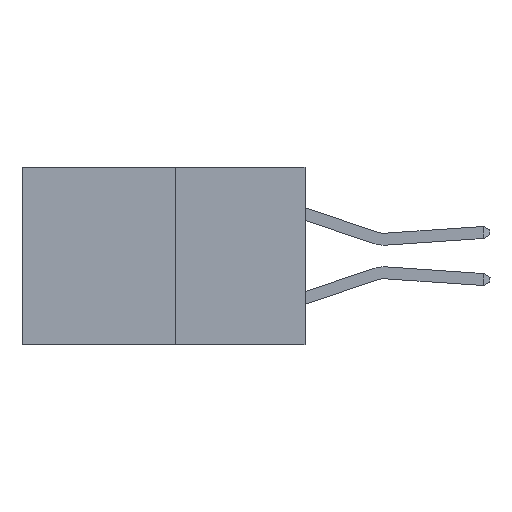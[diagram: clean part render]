
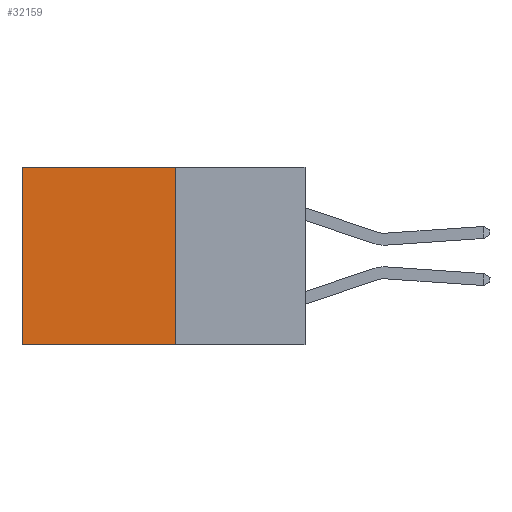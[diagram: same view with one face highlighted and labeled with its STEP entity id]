
A CAD part, left-side view. The second image highlights one B-rep face of the part: STEP entity #32159.
In plain terms, the highlighted planar face has unit normal (-1, 0, 0).
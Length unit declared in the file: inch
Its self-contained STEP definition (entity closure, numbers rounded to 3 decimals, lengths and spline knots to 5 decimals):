
#312 = EDGE_CURVE ( 'NONE', #10957, #1401, #4505, .T. ) ;
#1401 = VERTEX_POINT ( 'NONE', #15070 ) ;
#2053 = ORIENTED_EDGE ( 'NONE', *, *, #21790, .T. ) ;
#2580 = VECTOR ( 'NONE', #31204, 39.37008 ) ;
#4337 = LINE ( 'NONE', #11667, #10253 ) ;
#4505 = LINE ( 'NONE', #17044, #10426 ) ;
#4936 = VERTEX_POINT ( 'NONE', #7691 ) ;
#6424 = ORIENTED_EDGE ( 'NONE', *, *, #30421, .F. ) ;
#7115 = DIRECTION ( 'NONE',  ( 0., 0., -1. ) ) ;
#7643 = PLANE ( 'NONE',  #9791 ) ;
#7691 = CARTESIAN_POINT ( 'NONE',  ( 0.277, 0.59, -0.37 ) ) ;
#9660 = LINE ( 'NONE', #29312, #22921 ) ;
#9791 = AXIS2_PLACEMENT_3D ( 'NONE', #25100, #10161, #27577 ) ;
#10161 = DIRECTION ( 'NONE',  ( 1., 0., 0. ) ) ;
#10253 = VECTOR ( 'NONE', #14148, 39.37008 ) ;
#10426 = VECTOR ( 'NONE', #7115, 39.37008 ) ;
#10957 = VERTEX_POINT ( 'NONE', #26214 ) ;
#11667 = CARTESIAN_POINT ( 'NONE',  ( 0.277, 0.27, -0.37 ) ) ;
#14148 = DIRECTION ( 'NONE',  ( 0., 1., 0. ) ) ;
#14387 = DIRECTION ( 'NONE',  ( 0., 0., -1. ) ) ;
#15070 = CARTESIAN_POINT ( 'NONE',  ( 0.277, 0.27, -0.37 ) ) ;
#16068 = ORIENTED_EDGE ( 'NONE', *, *, #312, .F. ) ;
#17044 = CARTESIAN_POINT ( 'NONE',  ( 0.277, 0.27, -0.37 ) ) ;
#20658 = CARTESIAN_POINT ( 'NONE',  ( 0.277, 0.59, 0. ) ) ;
#21790 = EDGE_CURVE ( 'NONE', #10957, #29464, #22574, .T. ) ;
#22574 = LINE ( 'NONE', #28728, #2580 ) ;
#22921 = VECTOR ( 'NONE', #14387, 39.37008 ) ;
#23407 = FACE_OUTER_BOUND ( 'NONE', #25237, .T. ) ;
#25100 = CARTESIAN_POINT ( 'NONE',  ( 0.277, 0.27, -0.37 ) ) ;
#25237 = EDGE_LOOP ( 'NONE', ( #25770, #6424, #16068, #2053 ) ) ;
#25770 = ORIENTED_EDGE ( 'NONE', *, *, #27461, .T. ) ;
#26214 = CARTESIAN_POINT ( 'NONE',  ( 0.277, 0.27, 0. ) ) ;
#27461 = EDGE_CURVE ( 'NONE', #29464, #4936, #9660, .T. ) ;
#27577 = DIRECTION ( 'NONE',  ( 0., 0., -1. ) ) ;
#28728 = CARTESIAN_POINT ( 'NONE',  ( 0.277, 0.27, 0. ) ) ;
#29312 = CARTESIAN_POINT ( 'NONE',  ( 0.277, 0.59, -0.37 ) ) ;
#29464 = VERTEX_POINT ( 'NONE', #20658 ) ;
#30421 = EDGE_CURVE ( 'NONE', #1401, #4936, #4337, .T. ) ;
#31204 = DIRECTION ( 'NONE',  ( 0., 1., 0. ) ) ;
#32159 = ADVANCED_FACE ( 'NONE', ( #23407 ), #7643, .F. ) ;
